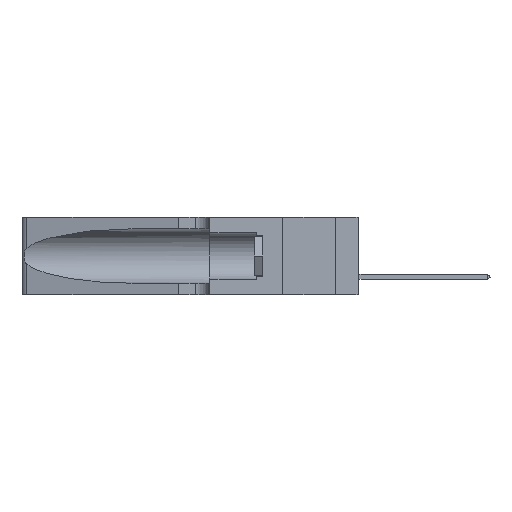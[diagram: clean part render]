
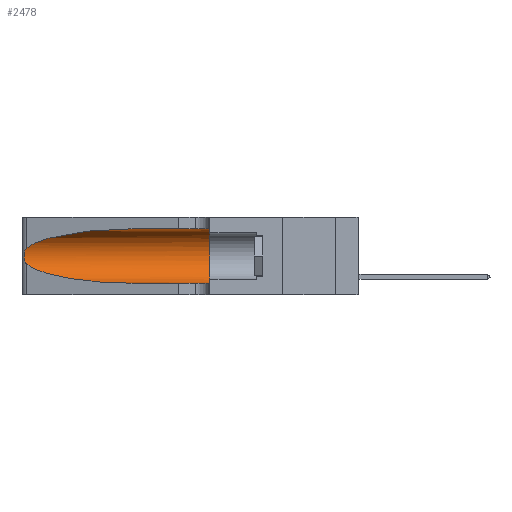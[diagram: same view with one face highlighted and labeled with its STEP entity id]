
A CAD part, left-side view. The second image highlights one B-rep face of the part: STEP entity #2478.
In plain terms, the highlighted cylindrical face has radius 3.308 mm (diameter 6.617 mm), a partial arc.
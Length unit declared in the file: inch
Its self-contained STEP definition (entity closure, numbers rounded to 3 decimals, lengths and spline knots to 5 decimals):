
#39 = CARTESIAN_POINT ( 'NONE',  ( 0.25487, 1.22718, 0.22369 ) ) ;
#167 =( BOUNDED_CURVE ( )  B_SPLINE_CURVE ( 3, ( #7721, #22702, #13903, #9864 ),
 .UNSPECIFIED., .F., .T. ) 
 B_SPLINE_CURVE_WITH_KNOTS ( ( 4, 4 ),
 ( 3.44316, 4.71239 ),
 .UNSPECIFIED. ) 
 CURVE ( )  GEOMETRIC_REPRESENTATION_ITEM ( )  RATIONAL_B_SPLINE_CURVE ( ( 1., 0.87, 0.87, 1. ) ) 
 REPRESENTATION_ITEM ( '' )  );
#627 = VERTEX_POINT ( 'NONE', #7418 ) ;
#2010 = CARTESIAN_POINT ( 'NONE',  ( 0.26018, 1.23835, 0.19895 ) ) ;
#2203 = CARTESIAN_POINT ( 'NONE',  ( 0.25555, 1.22993, 0.14849 ) ) ;
#2267 = VERTEX_POINT ( 'NONE', #17369 ) ;
#2478 = ADVANCED_FACE ( 'NONE', ( #5542 ), #21636, .F. ) ;
#2915 = VERTEX_POINT ( 'NONE', #20893 ) ;
#3774 = DIRECTION ( 'NONE',  ( 0., -1., 0. ) ) ;
#3862 = CARTESIAN_POINT ( 'NONE',  ( 0.25487, 1.22718, 0.22369 ) ) ;
#4163 = CARTESIAN_POINT ( 'NONE',  ( 0.25487, 1.22718, 0.14631 ) ) ;
#5532 = VECTOR ( 'NONE', #23353, 39.37008 ) ;
#5542 = FACE_OUTER_BOUND ( 'NONE', #12175, .T. ) ;
#6195 = DIRECTION ( 'NONE',  ( 0., 0., -1. ) ) ;
#6703 = EDGE_CURVE ( 'NONE', #627, #26177, #167, .T. ) ;
#6831 = DIRECTION ( 'NONE',  ( 0., 0., 1. ) ) ;
#7135 = CIRCLE ( 'NONE', #8638, 0.13025 ) ;
#7418 = CARTESIAN_POINT ( 'NONE',  ( 0.25487, 1.22718, 0.14631 ) ) ;
#7721 = CARTESIAN_POINT ( 'NONE',  ( 0.25487, 1.22718, 0.14631 ) ) ;
#8638 = AXIS2_PLACEMENT_3D ( 'NONE', #11125, #19592, #6831 ) ;
#9864 = CARTESIAN_POINT ( 'NONE',  ( 0.1305, 0.72297, 0.05475 ) ) ;
#10199 = CARTESIAN_POINT ( 'NONE',  ( 0.2373, 1.15595, 0.28018 ) ) ;
#10316 = EDGE_CURVE ( 'NONE', #21906, #2267, #18389, .T. ) ;
#10546 = ORIENTED_EDGE ( 'NONE', *, *, #15849, .T. ) ;
#10652 = CARTESIAN_POINT ( 'NONE',  ( 0.1305, 1.61858, 0.31525 ) ) ;
#11125 = CARTESIAN_POINT ( 'NONE',  ( 0.1305, 0.35, 0.185 ) ) ;
#11319 = ORIENTED_EDGE ( 'NONE', *, *, #10316, .F. ) ;
#12038 = CARTESIAN_POINT ( 'NONE',  ( 0.25487, 1.22718, 0.22369 ) ) ;
#12175 = EDGE_LOOP ( 'NONE', ( #13324, #10546, #16206, #23957, #22257, #11319 ) ) ;
#12191 = VERTEX_POINT ( 'NONE', #12038 ) ;
#12547 = LINE ( 'NONE', #23628, #5532 ) ;
#13030 = CARTESIAN_POINT ( 'NONE',  ( 0.26075, 1.23896, 0.19203 ) ) ;
#13324 = ORIENTED_EDGE ( 'NONE', *, *, #19734, .T. ) ;
#13903 = CARTESIAN_POINT ( 'NONE',  ( 0.18966, 0.96281, 0.05475 ) ) ;
#14355 = VECTOR ( 'NONE', #27553, 39.37008 ) ;
#14660 = EDGE_CURVE ( 'NONE', #26177, #2915, #12547, .T. ) ;
#14705 = CARTESIAN_POINT ( 'NONE',  ( 0.1305, 1.61858, 0.185 ) ) ;
#14784 = CARTESIAN_POINT ( 'NONE',  ( 0.25854, 1.2359, 0.20912 ) ) ;
#15081 = CARTESIAN_POINT ( 'NONE',  ( 0.25555, 1.22994, 0.2215 ) ) ;
#15849 = EDGE_CURVE ( 'NONE', #12191, #627, #16264, .T. ) ;
#16206 = ORIENTED_EDGE ( 'NONE', *, *, #6703, .T. ) ;
#16264 = B_SPLINE_CURVE_WITH_KNOTS ( 'NONE', 3,
 ( #39, #15081, #21475, #16960, #14784, #2010, #13030, #25873, #27758, #25592, #23612, #21562, #2203, #4163 ),
 .UNSPECIFIED., .F., .F.,
 ( 4, 2, 2, 2, 2, 2, 4 ),
 ( 0., 0.00027, 0.00053, 0.00107, 0.0016, 0.00187, 0.00214 ),
 .UNSPECIFIED. ) ;
#16680 = CARTESIAN_POINT ( 'NONE',  ( 0.1305, 0.72297, 0.31525 ) ) ;
#16737 = CARTESIAN_POINT ( 'NONE',  ( 0.1305, 0.72297, 0.05475 ) ) ;
#16960 = CARTESIAN_POINT ( 'NONE',  ( 0.25787, 1.23484, 0.2124 ) ) ;
#17369 = CARTESIAN_POINT ( 'NONE',  ( 0.1305, 0.35, 0.31525 ) ) ;
#18389 = LINE ( 'NONE', #10652, #14355 ) ;
#18541 = CARTESIAN_POINT ( 'NONE',  ( 0.18966, 0.96281, 0.31525 ) ) ;
#19592 = DIRECTION ( 'NONE',  ( 0., 1., 0. ) ) ;
#19734 = EDGE_CURVE ( 'NONE', #21906, #12191, #21770, .T. ) ;
#20893 = CARTESIAN_POINT ( 'NONE',  ( 0.1305, 0.35, 0.05475 ) ) ;
#21475 = CARTESIAN_POINT ( 'NONE',  ( 0.25639, 1.23184, 0.21858 ) ) ;
#21562 = CARTESIAN_POINT ( 'NONE',  ( 0.25639, 1.23186, 0.15144 ) ) ;
#21636 = CYLINDRICAL_SURFACE ( 'NONE', #27656, 0.13025 ) ;
#21770 =( BOUNDED_CURVE ( )  B_SPLINE_CURVE ( 3, ( #16680, #18541, #10199, #3862 ),
 .UNSPECIFIED., .F., .T. ) 
 B_SPLINE_CURVE_WITH_KNOTS ( ( 4, 4 ),
 ( 1.5708, 2.84003 ),
 .UNSPECIFIED. ) 
 CURVE ( )  GEOMETRIC_REPRESENTATION_ITEM ( )  RATIONAL_B_SPLINE_CURVE ( ( 1., 0.87, 0.87, 1. ) ) 
 REPRESENTATION_ITEM ( '' )  );
#21906 = VERTEX_POINT ( 'NONE', #24475 ) ;
#22257 = ORIENTED_EDGE ( 'NONE', *, *, #25245, .F. ) ;
#22702 = CARTESIAN_POINT ( 'NONE',  ( 0.2373, 1.15595, 0.08982 ) ) ;
#23353 = DIRECTION ( 'NONE',  ( 0., -1., 0. ) ) ;
#23612 = CARTESIAN_POINT ( 'NONE',  ( 0.25789, 1.23486, 0.15765 ) ) ;
#23628 = CARTESIAN_POINT ( 'NONE',  ( 0.1305, 1.61858, 0.05475 ) ) ;
#23957 = ORIENTED_EDGE ( 'NONE', *, *, #14660, .T. ) ;
#24475 = CARTESIAN_POINT ( 'NONE',  ( 0.1305, 0.72297, 0.31525 ) ) ;
#25245 = EDGE_CURVE ( 'NONE', #2267, #2915, #7135, .T. ) ;
#25592 = CARTESIAN_POINT ( 'NONE',  ( 0.25856, 1.23593, 0.16098 ) ) ;
#25873 = CARTESIAN_POINT ( 'NONE',  ( 0.26075, 1.23896, 0.178 ) ) ;
#26177 = VERTEX_POINT ( 'NONE', #16737 ) ;
#27553 = DIRECTION ( 'NONE',  ( 0., -1., 0. ) ) ;
#27656 = AXIS2_PLACEMENT_3D ( 'NONE', #14705, #3774, #6195 ) ;
#27758 = CARTESIAN_POINT ( 'NONE',  ( 0.26017, 1.23833, 0.17102 ) ) ;
